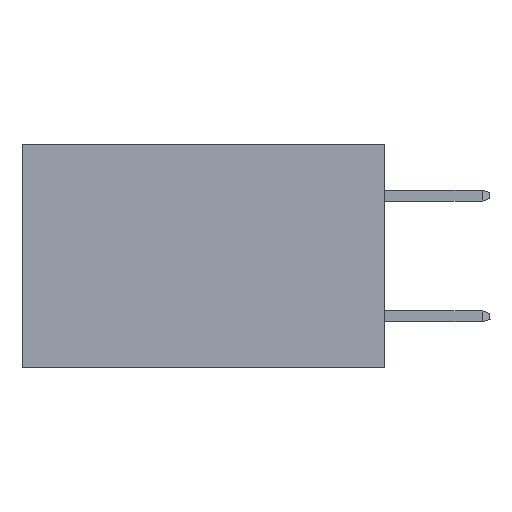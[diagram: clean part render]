
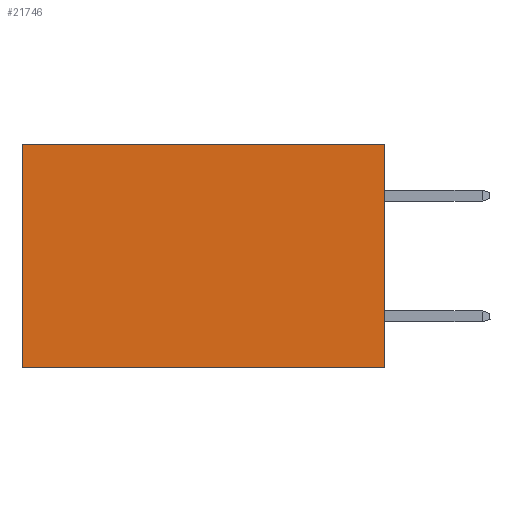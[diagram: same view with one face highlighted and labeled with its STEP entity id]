
A CAD part, left-side view. The second image highlights one B-rep face of the part: STEP entity #21746.
In plain terms, the highlighted planar face has unit normal (-1, 0, 0).
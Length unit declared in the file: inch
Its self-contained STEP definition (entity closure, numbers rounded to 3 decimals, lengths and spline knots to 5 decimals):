
#615 = DIRECTION ( 'NONE',  ( 0., 1., 0. ) ) ;
#970 = LINE ( 'NONE', #24721, #1612 ) ;
#1612 = VECTOR ( 'NONE', #14885, 39.37008 ) ;
#1770 = ORIENTED_EDGE ( 'NONE', *, *, #7980, .T. ) ;
#2655 = CARTESIAN_POINT ( 'NONE',  ( 0.2615, 0., -0.37 ) ) ;
#3163 = EDGE_CURVE ( 'NONE', #10322, #12910, #11086, .T. ) ;
#3713 = ORIENTED_EDGE ( 'NONE', *, *, #3163, .F. ) ;
#6293 = ORIENTED_EDGE ( 'NONE', *, *, #10083, .F. ) ;
#6465 = CARTESIAN_POINT ( 'NONE',  ( 0.2615, 0., 0. ) ) ;
#7111 = DIRECTION ( 'NONE',  ( 0., 0., -1. ) ) ;
#7269 = CARTESIAN_POINT ( 'NONE',  ( 0.2615, 0., -0.37 ) ) ;
#7980 = EDGE_CURVE ( 'NONE', #9162, #21347, #970, .T. ) ;
#8544 = DIRECTION ( 'NONE',  ( 0., 1., 0. ) ) ;
#9162 = VERTEX_POINT ( 'NONE', #24092 ) ;
#9595 = CARTESIAN_POINT ( 'NONE',  ( 0.2615, 0., -0.37 ) ) ;
#10041 = DIRECTION ( 'NONE',  ( 1., 0., 0. ) ) ;
#10083 = EDGE_CURVE ( 'NONE', #12910, #21347, #11212, .T. ) ;
#10322 = VERTEX_POINT ( 'NONE', #23615 ) ;
#10584 = EDGE_CURVE ( 'NONE', #10322, #9162, #15194, .T. ) ;
#11086 = LINE ( 'NONE', #7269, #20953 ) ;
#11212 = LINE ( 'NONE', #2655, #21080 ) ;
#11935 = PLANE ( 'NONE',  #24868 ) ;
#12910 = VERTEX_POINT ( 'NONE', #9595 ) ;
#14215 = EDGE_LOOP ( 'NONE', ( #1770, #6293, #3713, #14795 ) ) ;
#14795 = ORIENTED_EDGE ( 'NONE', *, *, #10584, .T. ) ;
#14885 = DIRECTION ( 'NONE',  ( 0., 0., -1. ) ) ;
#15194 = LINE ( 'NONE', #6465, #19824 ) ;
#19824 = VECTOR ( 'NONE', #8544, 39.37008 ) ;
#20953 = VECTOR ( 'NONE', #7111, 39.37008 ) ;
#21080 = VECTOR ( 'NONE', #615, 39.37008 ) ;
#21347 = VERTEX_POINT ( 'NONE', #22726 ) ;
#21746 = ADVANCED_FACE ( 'NONE', ( #22412 ), #11935, .F. ) ;
#21862 = CARTESIAN_POINT ( 'NONE',  ( 0.2615, 0., -0.37 ) ) ;
#22412 = FACE_OUTER_BOUND ( 'NONE', #14215, .T. ) ;
#22726 = CARTESIAN_POINT ( 'NONE',  ( 0.2615, 0.6, -0.37 ) ) ;
#23615 = CARTESIAN_POINT ( 'NONE',  ( 0.2615, 0., 0. ) ) ;
#23856 = DIRECTION ( 'NONE',  ( 0., 0., -1. ) ) ;
#24092 = CARTESIAN_POINT ( 'NONE',  ( 0.2615, 0.6, 0. ) ) ;
#24721 = CARTESIAN_POINT ( 'NONE',  ( 0.2615, 0.6, -0.37 ) ) ;
#24868 = AXIS2_PLACEMENT_3D ( 'NONE', #21862, #10041, #23856 ) ;
